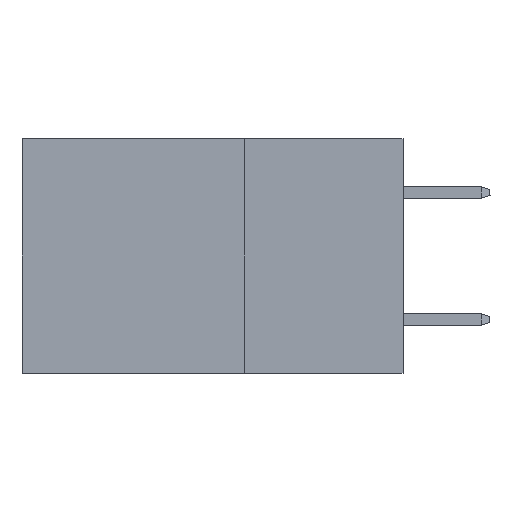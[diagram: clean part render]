
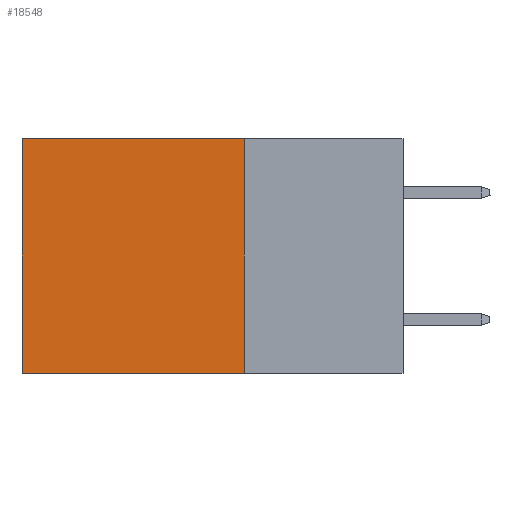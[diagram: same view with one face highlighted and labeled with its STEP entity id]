
A CAD part, left-side view. The second image highlights one B-rep face of the part: STEP entity #18548.
In plain terms, the highlighted planar face has unit normal (-1, 0, 0).
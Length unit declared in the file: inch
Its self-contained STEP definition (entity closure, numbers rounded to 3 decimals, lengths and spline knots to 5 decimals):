
#772 = ORIENTED_EDGE ( 'NONE', *, *, #16740, .T. ) ;
#1204 = VERTEX_POINT ( 'NONE', #3802 ) ;
#1411 = FACE_OUTER_BOUND ( 'NONE', #24270, .T. ) ;
#1720 = EDGE_CURVE ( 'NONE', #1204, #24177, #12186, .T. ) ;
#2083 = LINE ( 'NONE', #23660, #14881 ) ;
#2633 = EDGE_CURVE ( 'NONE', #3948, #24177, #2083, .T. ) ;
#3802 = CARTESIAN_POINT ( 'NONE',  ( 0.2875, 0.25, -0.37 ) ) ;
#3948 = VERTEX_POINT ( 'NONE', #13661 ) ;
#5518 = EDGE_CURVE ( 'NONE', #27181, #1204, #16707, .T. ) ;
#9669 = DIRECTION ( 'NONE',  ( 1., 0., 0. ) ) ;
#12186 = LINE ( 'NONE', #25883, #19371 ) ;
#12251 = VECTOR ( 'NONE', #19690, 39.37008 ) ;
#12314 = PLANE ( 'NONE',  #13062 ) ;
#13062 = AXIS2_PLACEMENT_3D ( 'NONE', #22979, #9669, #33718 ) ;
#13661 = CARTESIAN_POINT ( 'NONE',  ( 0.2875, 0.6, 0. ) ) ;
#13976 = CARTESIAN_POINT ( 'NONE',  ( 0.2875, 0.25, 0. ) ) ;
#14680 = VECTOR ( 'NONE', #24815, 39.37008 ) ;
#14691 = ORIENTED_EDGE ( 'NONE', *, *, #5518, .F. ) ;
#14881 = VECTOR ( 'NONE', #29121, 39.37008 ) ;
#15079 = CARTESIAN_POINT ( 'NONE',  ( 0.2875, 0.6, -0.37 ) ) ;
#16707 = LINE ( 'NONE', #22546, #12251 ) ;
#16740 = EDGE_CURVE ( 'NONE', #27181, #3948, #29905, .T. ) ;
#17127 = CARTESIAN_POINT ( 'NONE',  ( 0.2875, 0.25, 0. ) ) ;
#18548 = ADVANCED_FACE ( 'NONE', ( #1411 ), #12314, .F. ) ;
#19371 = VECTOR ( 'NONE', #23035, 39.37008 ) ;
#19690 = DIRECTION ( 'NONE',  ( 0., 0., -1. ) ) ;
#22546 = CARTESIAN_POINT ( 'NONE',  ( 0.2875, 0.25, 0. ) ) ;
#22979 = CARTESIAN_POINT ( 'NONE',  ( 0.2875, 0.25, 0. ) ) ;
#23035 = DIRECTION ( 'NONE',  ( 0., 1., 0. ) ) ;
#23660 = CARTESIAN_POINT ( 'NONE',  ( 0.2875, 0.6, 0. ) ) ;
#24177 = VERTEX_POINT ( 'NONE', #15079 ) ;
#24270 = EDGE_LOOP ( 'NONE', ( #26151, #31051, #14691, #772 ) ) ;
#24815 = DIRECTION ( 'NONE',  ( 0., 1., 0. ) ) ;
#25883 = CARTESIAN_POINT ( 'NONE',  ( 0.2875, 0.25, -0.37 ) ) ;
#26151 = ORIENTED_EDGE ( 'NONE', *, *, #2633, .T. ) ;
#27181 = VERTEX_POINT ( 'NONE', #17127 ) ;
#29121 = DIRECTION ( 'NONE',  ( 0., 0., -1. ) ) ;
#29905 = LINE ( 'NONE', #13976, #14680 ) ;
#31051 = ORIENTED_EDGE ( 'NONE', *, *, #1720, .F. ) ;
#33718 = DIRECTION ( 'NONE',  ( 0., 0., -1. ) ) ;
